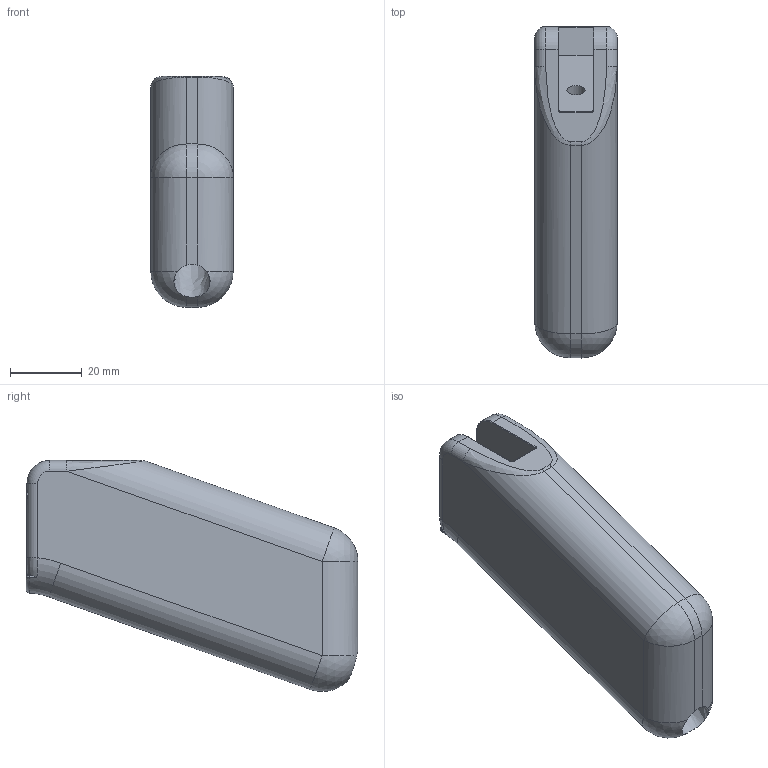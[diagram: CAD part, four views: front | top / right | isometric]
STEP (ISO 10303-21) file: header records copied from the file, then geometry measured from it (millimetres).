
FILE_DESCRIPTION (( 'STEP AP214' ), '1' );
FILE_NAME ('Smooth_AR_Grip.STEP', '2014-02-17T06:48:20', ( 'elpi' ), ( '' ), 'SwSTEP 2.0', 'SolidWorks 2013', '' );
FILE_SCHEMA (( 'AUTOMOTIVE_DESIGN' ));
Length unit declared in the file: millimetre
Products named in the file (1): Smooth_AR_Grip
Bounding box: 23.02 x 92.72 x 64.56 mm (x, y, z)
Volume: 75323.9 mm3; surface area: 16074.2 mm2
Topology: 1 solids, 1 shells, 81 faces, 200 edges, 119 vertices
Faces by surface type: cylinder 29, bspline 21, plane 19, torus 8, sphere 4
Full cylindrical faces by diameter (mm): 3.429 x1, 5.105 x1
Entity records: 3728 total; most frequent: CARTESIAN_POINT 2022, ORIENTED_EDGE 384, DIRECTION 293, EDGE_CURVE 192, VERTEX_POINT 117, AXIS2_PLACEMENT_3D 116, EDGE_LOOP 87, FACE_OUTER_BOUND 85
